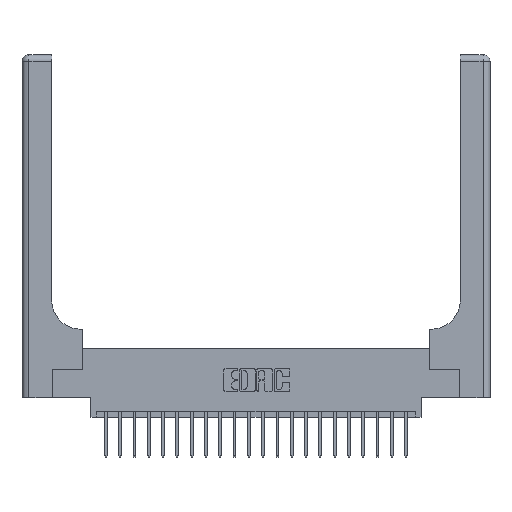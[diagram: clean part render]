
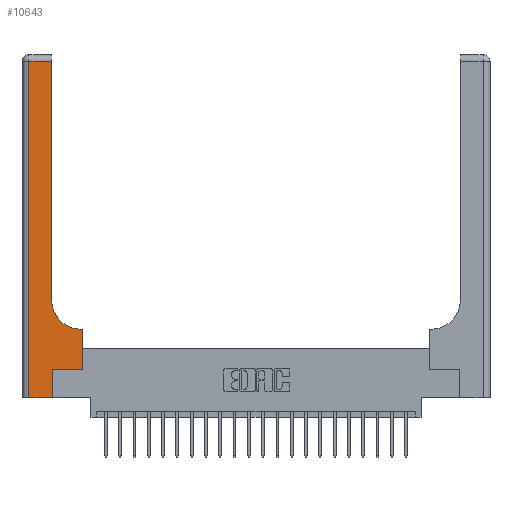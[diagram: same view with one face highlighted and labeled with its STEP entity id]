
A CAD part, top view. The second image highlights one B-rep face of the part: STEP entity #10643.
In plain terms, the highlighted planar face has unit normal (0, 0, 1).
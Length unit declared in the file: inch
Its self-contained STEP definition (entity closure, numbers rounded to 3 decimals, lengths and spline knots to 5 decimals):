
#27 = DIRECTION ( 'NONE',  ( -1., 0., 0. ) ) ;
#200 = VECTOR ( 'NONE', #11562, 39.37008 ) ;
#408 = EDGE_CURVE ( 'NONE', #21432, #13713, #19606, .T. ) ;
#515 = EDGE_CURVE ( 'NONE', #4229, #22241, #878, .T. ) ;
#545 = EDGE_LOOP ( 'NONE', ( #1240, #16018, #17410, #11283, #10667, #15471, #20653, #9798, #20972 ) ) ;
#712 = EDGE_CURVE ( 'NONE', #13713, #7549, #17824, .T. ) ;
#878 = LINE ( 'NONE', #13861, #1129 ) ;
#916 = LINE ( 'NONE', #11761, #3931 ) ;
#1129 = VECTOR ( 'NONE', #20936, 39.37008 ) ;
#1240 = ORIENTED_EDGE ( 'NONE', *, *, #515, .T. ) ;
#1335 = VERTEX_POINT ( 'NONE', #9567 ) ;
#2710 = CARTESIAN_POINT ( 'NONE',  ( 0., 0., 0.37 ) ) ;
#3734 = CARTESIAN_POINT ( 'NONE',  ( 0.265, 0.25, 0.37 ) ) ;
#3746 = EDGE_CURVE ( 'NONE', #1335, #20196, #916, .T. ) ;
#3763 = LINE ( 'NONE', #10767, #5339 ) ;
#3931 = VECTOR ( 'NONE', #4516, 39.37008 ) ;
#4146 = CARTESIAN_POINT ( 'NONE',  ( 0.528, 0.25, 0.37 ) ) ;
#4229 = VERTEX_POINT ( 'NONE', #16590 ) ;
#4516 = DIRECTION ( 'NONE',  ( 0., 1., 0. ) ) ;
#4765 = LINE ( 'NONE', #2710, #200 ) ;
#4893 = CARTESIAN_POINT ( 'NONE',  ( 0.06, 0., 0.37 ) ) ;
#5339 = VECTOR ( 'NONE', #14330, 39.37008 ) ;
#5484 = AXIS2_PLACEMENT_3D ( 'NONE', #8168, #22143, #15422 ) ;
#5945 = EDGE_CURVE ( 'NONE', #7549, #4229, #21540, .T. ) ;
#6780 = EDGE_CURVE ( 'NONE', #22241, #22003, #17448, .T. ) ;
#6966 = CARTESIAN_POINT ( 'NONE',  ( 0.51, 0.6, 0.37 ) ) ;
#7549 = VERTEX_POINT ( 'NONE', #6966 ) ;
#7714 = EDGE_CURVE ( 'NONE', #22003, #16536, #3763, .T. ) ;
#8168 = CARTESIAN_POINT ( 'NONE',  ( 0., 3., 0.37 ) ) ;
#8411 = VECTOR ( 'NONE', #20529, 39.37008 ) ;
#9051 = EDGE_CURVE ( 'NONE', #16536, #1335, #4765, .T. ) ;
#9567 = CARTESIAN_POINT ( 'NONE',  ( 0.265, 0., 0.37 ) ) ;
#9776 = PLANE ( 'NONE',  #5484 ) ;
#9798 = ORIENTED_EDGE ( 'NONE', *, *, #712, .T. ) ;
#10005 = CARTESIAN_POINT ( 'NONE',  ( 0.265, 0.25, 0.37 ) ) ;
#10643 = ADVANCED_FACE ( 'NONE', ( #18462 ), #9776, .F. ) ;
#10667 = ORIENTED_EDGE ( 'NONE', *, *, #3746, .T. ) ;
#10741 = EDGE_CURVE ( 'NONE', #20196, #21432, #20192, .T. ) ;
#10767 = CARTESIAN_POINT ( 'NONE',  ( 0.06, 3., 0.37 ) ) ;
#11082 = CARTESIAN_POINT ( 'NONE',  ( 0.528, 0.6, 0.37 ) ) ;
#11283 = ORIENTED_EDGE ( 'NONE', *, *, #9051, .T. ) ;
#11562 = DIRECTION ( 'NONE',  ( 1., 0., 0. ) ) ;
#11761 = CARTESIAN_POINT ( 'NONE',  ( 0.265, 0., 0.37 ) ) ;
#12006 = CARTESIAN_POINT ( 'NONE',  ( 0., 2.94, 0.37 ) ) ;
#13713 = VERTEX_POINT ( 'NONE', #11082 ) ;
#13861 = CARTESIAN_POINT ( 'NONE',  ( 0.26, 3., 0.37 ) ) ;
#13983 = CARTESIAN_POINT ( 'NONE',  ( 0.26, 0.6, 0.37 ) ) ;
#14330 = DIRECTION ( 'NONE',  ( 0., -1., 0. ) ) ;
#15401 = DIRECTION ( 'NONE',  ( 0., 0., -1. ) ) ;
#15422 = DIRECTION ( 'NONE',  ( -1., 0., 0. ) ) ;
#15471 = ORIENTED_EDGE ( 'NONE', *, *, #10741, .T. ) ;
#15722 = VECTOR ( 'NONE', #27, 39.37008 ) ;
#16018 = ORIENTED_EDGE ( 'NONE', *, *, #6780, .T. ) ;
#16233 = DIRECTION ( 'NONE',  ( 0., 1., 0. ) ) ;
#16536 = VERTEX_POINT ( 'NONE', #4893 ) ;
#16590 = CARTESIAN_POINT ( 'NONE',  ( 0.26, 0.85, 0.37 ) ) ;
#16808 = CARTESIAN_POINT ( 'NONE',  ( 0.51, 0.85, 0.37 ) ) ;
#17106 = CARTESIAN_POINT ( 'NONE',  ( 0.06, 2.94, 0.37 ) ) ;
#17211 = CARTESIAN_POINT ( 'NONE',  ( 0.528, 0.25, 0.37 ) ) ;
#17410 = ORIENTED_EDGE ( 'NONE', *, *, #7714, .T. ) ;
#17448 = LINE ( 'NONE', #12006, #21122 ) ;
#17824 = LINE ( 'NONE', #13983, #15722 ) ;
#18024 = VECTOR ( 'NONE', #16233, 39.37008 ) ;
#18462 = FACE_OUTER_BOUND ( 'NONE', #545, .T. ) ;
#18602 = AXIS2_PLACEMENT_3D ( 'NONE', #16808, #15401, #18790 ) ;
#18790 = DIRECTION ( 'NONE',  ( 1., 0., 0. ) ) ;
#19169 = DIRECTION ( 'NONE',  ( -1., 0., 0. ) ) ;
#19606 = LINE ( 'NONE', #4146, #18024 ) ;
#20192 = LINE ( 'NONE', #10005, #8411 ) ;
#20196 = VERTEX_POINT ( 'NONE', #3734 ) ;
#20529 = DIRECTION ( 'NONE',  ( 1., 0., 0. ) ) ;
#20653 = ORIENTED_EDGE ( 'NONE', *, *, #408, .T. ) ;
#20936 = DIRECTION ( 'NONE',  ( 0., 1., 0. ) ) ;
#20972 = ORIENTED_EDGE ( 'NONE', *, *, #5945, .T. ) ;
#21122 = VECTOR ( 'NONE', #19169, 39.37008 ) ;
#21432 = VERTEX_POINT ( 'NONE', #17211 ) ;
#21540 = CIRCLE ( 'NONE', #18602, 0.25 ) ;
#21828 = CARTESIAN_POINT ( 'NONE',  ( 0.26, 2.94, 0.37 ) ) ;
#22003 = VERTEX_POINT ( 'NONE', #17106 ) ;
#22143 = DIRECTION ( 'NONE',  ( 0., 0., -1. ) ) ;
#22241 = VERTEX_POINT ( 'NONE', #21828 ) ;
